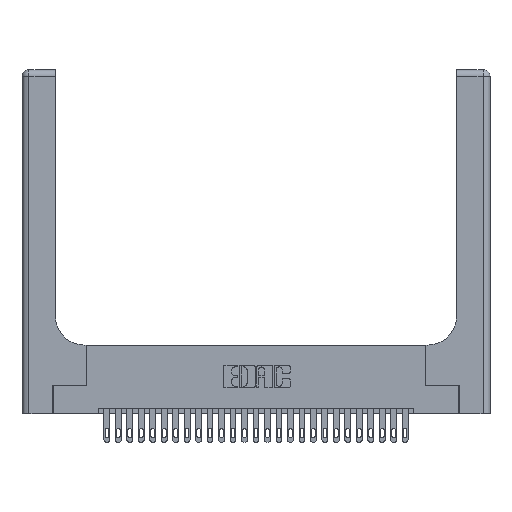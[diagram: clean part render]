
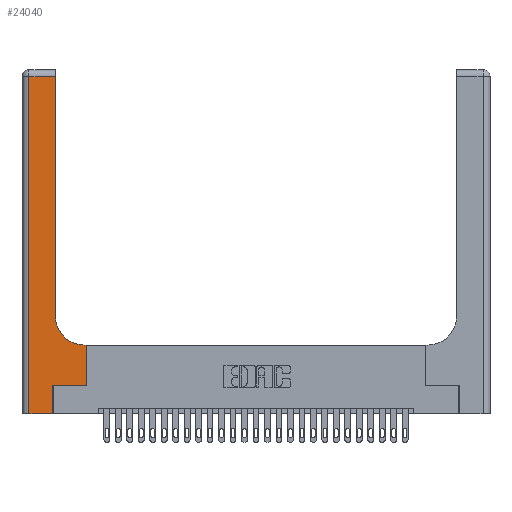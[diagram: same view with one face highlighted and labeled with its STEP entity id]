
A CAD part, top view. The second image highlights one B-rep face of the part: STEP entity #24040.
In plain terms, the highlighted planar face has unit normal (0, 0, 1).
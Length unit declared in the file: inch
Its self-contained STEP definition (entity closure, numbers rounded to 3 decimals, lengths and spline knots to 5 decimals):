
#49 = VERTEX_POINT ( 'NONE', #4879 ) ;
#142 = CARTESIAN_POINT ( 'NONE',  ( 0.06, 0., 0.37 ) ) ;
#761 = EDGE_CURVE ( 'NONE', #18346, #1861, #1979, .T. ) ;
#1717 = CARTESIAN_POINT ( 'NONE',  ( 0.269, 0., 0.37 ) ) ;
#1825 = CARTESIAN_POINT ( 'NONE',  ( 0.5415, 0.6, 0.37 ) ) ;
#1861 = VERTEX_POINT ( 'NONE', #14963 ) ;
#1972 = CARTESIAN_POINT ( 'NONE',  ( 0.2915, 0.6, 0.37 ) ) ;
#1979 = LINE ( 'NONE', #5725, #5739 ) ;
#2548 = LINE ( 'NONE', #1717, #21441 ) ;
#2616 = VERTEX_POINT ( 'NONE', #5543 ) ;
#3239 = DIRECTION ( 'NONE',  ( 0., 0., -1. ) ) ;
#3314 = VECTOR ( 'NONE', #27000, 39.37008 ) ;
#4140 = VERTEX_POINT ( 'NONE', #14645 ) ;
#4156 = CARTESIAN_POINT ( 'NONE',  ( 0.5585, 0.25, 0.37 ) ) ;
#4879 = CARTESIAN_POINT ( 'NONE',  ( 0.5585, 0.6, 0.37 ) ) ;
#5203 = ORIENTED_EDGE ( 'NONE', *, *, #7637, .T. ) ;
#5543 = CARTESIAN_POINT ( 'NONE',  ( 0.06, 2.94, 0.37 ) ) ;
#5725 = CARTESIAN_POINT ( 'NONE',  ( 0., 0., 0.37 ) ) ;
#5739 = VECTOR ( 'NONE', #27834, 39.37008 ) ;
#5889 = DIRECTION ( 'NONE',  ( 0., 0., -1. ) ) ;
#6348 = EDGE_CURVE ( 'NONE', #49, #23812, #23865, .T. ) ;
#6418 = DIRECTION ( 'NONE',  ( 0., 1., 0. ) ) ;
#6457 = LINE ( 'NONE', #10990, #19510 ) ;
#6712 = ORIENTED_EDGE ( 'NONE', *, *, #13852, .T. ) ;
#7027 = VERTEX_POINT ( 'NONE', #14969 ) ;
#7398 = VECTOR ( 'NONE', #6418, 39.37008 ) ;
#7490 = ORIENTED_EDGE ( 'NONE', *, *, #23337, .T. ) ;
#7494 = ORIENTED_EDGE ( 'NONE', *, *, #9041, .T. ) ;
#7637 = EDGE_CURVE ( 'NONE', #1861, #4140, #2548, .T. ) ;
#8717 = VERTEX_POINT ( 'NONE', #11388 ) ;
#9041 = EDGE_CURVE ( 'NONE', #16075, #2616, #25110, .T. ) ;
#9455 = LINE ( 'NONE', #4156, #7398 ) ;
#9688 = CIRCLE ( 'NONE', #25557, 0.25 ) ;
#10572 = ORIENTED_EDGE ( 'NONE', *, *, #761, .T. ) ;
#10764 = ORIENTED_EDGE ( 'NONE', *, *, #22835, .T. ) ;
#10990 = CARTESIAN_POINT ( 'NONE',  ( 0.06, 3., 0.37 ) ) ;
#11225 = CARTESIAN_POINT ( 'NONE',  ( 0., 2.94, 0.37 ) ) ;
#11305 = ORIENTED_EDGE ( 'NONE', *, *, #18730, .T. ) ;
#11388 = CARTESIAN_POINT ( 'NONE',  ( 0.2915, 0.85, 0.37 ) ) ;
#11663 = AXIS2_PLACEMENT_3D ( 'NONE', #11970, #3239, #24990 ) ;
#11970 = CARTESIAN_POINT ( 'NONE',  ( 0., 3., 0.37 ) ) ;
#12435 = CARTESIAN_POINT ( 'NONE',  ( 0.5415, 0.85, 0.37 ) ) ;
#12744 = VECTOR ( 'NONE', #15589, 39.37008 ) ;
#13032 = DIRECTION ( 'NONE',  ( -1., 0., 0. ) ) ;
#13732 = FACE_OUTER_BOUND ( 'NONE', #21666, .T. ) ;
#13852 = EDGE_CURVE ( 'NONE', #7027, #49, #9455, .T. ) ;
#14645 = CARTESIAN_POINT ( 'NONE',  ( 0.269, 0.25, 0.37 ) ) ;
#14790 = DIRECTION ( 'NONE',  ( 0., 1., 0. ) ) ;
#14963 = CARTESIAN_POINT ( 'NONE',  ( 0.269, 0., 0.37 ) ) ;
#14969 = CARTESIAN_POINT ( 'NONE',  ( 0.5585, 0.25, 0.37 ) ) ;
#15311 = VECTOR ( 'NONE', #19617, 39.37008 ) ;
#15589 = DIRECTION ( 'NONE',  ( 0., 1., 0. ) ) ;
#16075 = VERTEX_POINT ( 'NONE', #18512 ) ;
#18346 = VERTEX_POINT ( 'NONE', #142 ) ;
#18512 = CARTESIAN_POINT ( 'NONE',  ( 0.2915, 2.94, 0.37 ) ) ;
#18730 = EDGE_CURVE ( 'NONE', #23812, #8717, #9688, .T. ) ;
#19510 = VECTOR ( 'NONE', #26294, 39.37008 ) ;
#19617 = DIRECTION ( 'NONE',  ( -1., 0., 0. ) ) ;
#19778 = ORIENTED_EDGE ( 'NONE', *, *, #24499, .T. ) ;
#20612 = PLANE ( 'NONE',  #11663 ) ;
#20645 = LINE ( 'NONE', #26468, #12744 ) ;
#20990 = DIRECTION ( 'NONE',  ( 1., 0., 0. ) ) ;
#21441 = VECTOR ( 'NONE', #14790, 39.37008 ) ;
#21666 = EDGE_LOOP ( 'NONE', ( #7490, #7494, #19778, #10572, #5203, #10764, #6712, #28133, #11305 ) ) ;
#22014 = VECTOR ( 'NONE', #13032, 39.37008 ) ;
#22163 = LINE ( 'NONE', #24515, #3314 ) ;
#22835 = EDGE_CURVE ( 'NONE', #4140, #7027, #22163, .T. ) ;
#23337 = EDGE_CURVE ( 'NONE', #8717, #16075, #20645, .T. ) ;
#23812 = VERTEX_POINT ( 'NONE', #1825 ) ;
#23865 = LINE ( 'NONE', #1972, #15311 ) ;
#24040 = ADVANCED_FACE ( 'NONE', ( #13732 ), #20612, .F. ) ;
#24499 = EDGE_CURVE ( 'NONE', #2616, #18346, #6457, .T. ) ;
#24515 = CARTESIAN_POINT ( 'NONE',  ( 0.269, 0.25, 0.37 ) ) ;
#24990 = DIRECTION ( 'NONE',  ( -1., 0., 0. ) ) ;
#25110 = LINE ( 'NONE', #11225, #22014 ) ;
#25557 = AXIS2_PLACEMENT_3D ( 'NONE', #12435, #5889, #20990 ) ;
#26294 = DIRECTION ( 'NONE',  ( 0., -1., 0. ) ) ;
#26468 = CARTESIAN_POINT ( 'NONE',  ( 0.2915, 3., 0.37 ) ) ;
#27000 = DIRECTION ( 'NONE',  ( 1., 0., 0. ) ) ;
#27834 = DIRECTION ( 'NONE',  ( 1., 0., 0. ) ) ;
#28133 = ORIENTED_EDGE ( 'NONE', *, *, #6348, .T. ) ;
